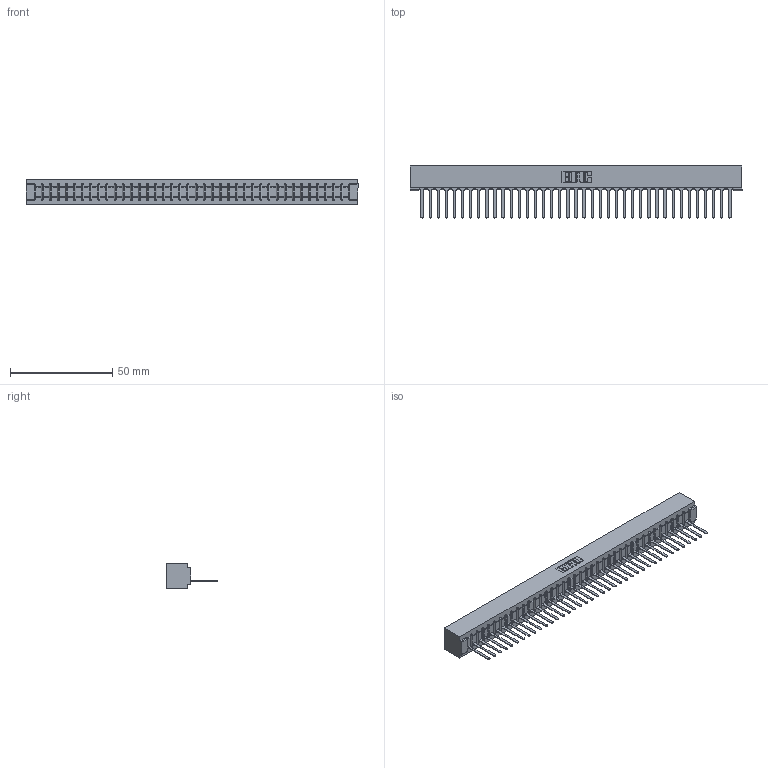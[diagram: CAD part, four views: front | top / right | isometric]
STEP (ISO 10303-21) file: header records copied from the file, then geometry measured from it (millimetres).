
FILE_DESCRIPTION (( 'STEP AP203' ), '1' );
FILE_NAME ('307-039-447-101.STEP', '2020-09-29T07:37:23', ( '' ), ( '' ), 'SwSTEP 2.0', 'SolidWorks 2020', '' );
FILE_SCHEMA (( 'CONFIG_CONTROL_DESIGN' ));
Length unit declared in the file: inch
Products named in the file (3): 307-290-001_547; 307 Part_No Mounting Lugs; 307-039-447-101
Assembly tree (40 placements, depth 2):
  307-039-447-101
    307 Part_No Mounting Lugs
    307-290-001_547  x39
Bounding box: 162.41 x 25.43 x 12.7 mm (x, y, z)
Volume: 17442.2 mm3; surface area: 19143.2 mm2
Topology: 40 solids, 40 shells, 2334 faces, 6617 edges, 4250 vertices
Faces by surface type: plane 1509, cylinder 745, sphere 80
Entity records: 33494 total; most frequent: CARTESIAN_POINT 5640, ORIENTED_EDGE 5626, DIRECTION 5485, EDGE_CURVE 2813, VECTOR 2159, LINE 2159, VERTEX_POINT 1818, AXIS2_PLACEMENT_3D 1663
